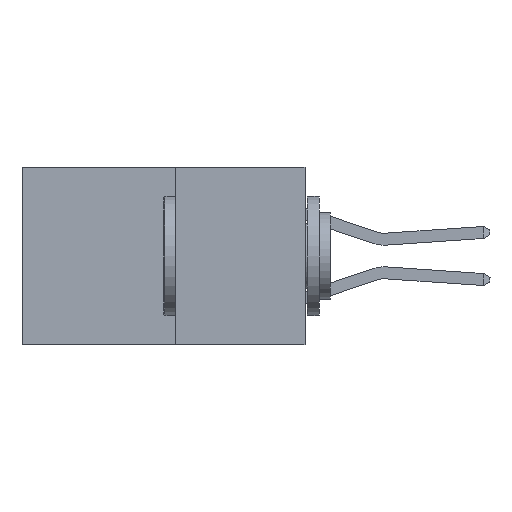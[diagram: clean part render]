
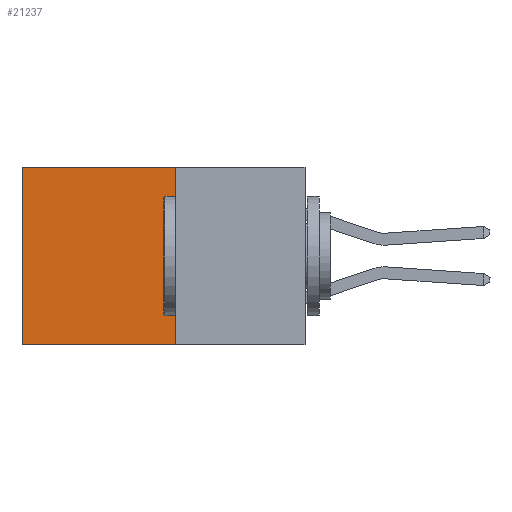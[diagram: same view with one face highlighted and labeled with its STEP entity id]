
A CAD part, left-side view. The second image highlights one B-rep face of the part: STEP entity #21237.
In plain terms, the highlighted planar face has unit normal (-1, 0, 0).
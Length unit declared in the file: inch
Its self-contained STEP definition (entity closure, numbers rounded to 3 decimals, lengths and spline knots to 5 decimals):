
#1875 = ORIENTED_EDGE ( 'NONE', *, *, #5821, .T. ) ;
#1978 = DIRECTION ( 'NONE',  ( 0., 1., 0. ) ) ;
#2347 = CARTESIAN_POINT ( 'NONE',  ( 0.277, 0.59, -0.37 ) ) ;
#3341 = CARTESIAN_POINT ( 'NONE',  ( 0.277, 0.27, -0.37 ) ) ;
#3669 = VECTOR ( 'NONE', #21332, 39.37008 ) ;
#4539 = CARTESIAN_POINT ( 'NONE',  ( 0.277, 0.27, 0. ) ) ;
#5821 = EDGE_CURVE ( 'NONE', #18430, #14609, #11507, .T. ) ;
#5999 = CARTESIAN_POINT ( 'NONE',  ( 0.277, 0.27, -0.37 ) ) ;
#6032 = CARTESIAN_POINT ( 'NONE',  ( 0.277, 0.27, 0. ) ) ;
#7014 = FACE_OUTER_BOUND ( 'NONE', #12548, .T. ) ;
#8578 = PLANE ( 'NONE',  #15461 ) ;
#10175 = ORIENTED_EDGE ( 'NONE', *, *, #31992, .F. ) ;
#10343 = DIRECTION ( 'NONE',  ( 0., 0., -1. ) ) ;
#10533 = CARTESIAN_POINT ( 'NONE',  ( 0.277, 0.59, -0.37 ) ) ;
#10914 = ORIENTED_EDGE ( 'NONE', *, *, #27633, .T. ) ;
#11176 = DIRECTION ( 'NONE',  ( 0., 0., -1. ) ) ;
#11507 = LINE ( 'NONE', #10533, #12329 ) ;
#12329 = VECTOR ( 'NONE', #10343, 39.37008 ) ;
#12548 = EDGE_LOOP ( 'NONE', ( #1875, #32816, #10175, #10914 ) ) ;
#12739 = DIRECTION ( 'NONE',  ( 0., 0., -1. ) ) ;
#13264 = VECTOR ( 'NONE', #1978, 39.37008 ) ;
#14609 = VERTEX_POINT ( 'NONE', #2347 ) ;
#15461 = AXIS2_PLACEMENT_3D ( 'NONE', #5999, #16242, #11176 ) ;
#16242 = DIRECTION ( 'NONE',  ( 1., 0., 0. ) ) ;
#18430 = VERTEX_POINT ( 'NONE', #27172 ) ;
#21237 = ADVANCED_FACE ( 'NONE', ( #7014 ), #8578, .F. ) ;
#21332 = DIRECTION ( 'NONE',  ( 0., 1., 0. ) ) ;
#22663 = VERTEX_POINT ( 'NONE', #6032 ) ;
#23397 = LINE ( 'NONE', #3341, #3669 ) ;
#25602 = CARTESIAN_POINT ( 'NONE',  ( 0.277, 0.27, -0.37 ) ) ;
#25870 = CARTESIAN_POINT ( 'NONE',  ( 0.277, 0.27, -0.37 ) ) ;
#26308 = LINE ( 'NONE', #25602, #32348 ) ;
#26997 = LINE ( 'NONE', #4539, #13264 ) ;
#27172 = CARTESIAN_POINT ( 'NONE',  ( 0.277, 0.59, 0. ) ) ;
#27633 = EDGE_CURVE ( 'NONE', #22663, #18430, #26997, .T. ) ;
#28521 = VERTEX_POINT ( 'NONE', #25870 ) ;
#31992 = EDGE_CURVE ( 'NONE', #22663, #28521, #26308, .T. ) ;
#32348 = VECTOR ( 'NONE', #12739, 39.37008 ) ;
#32816 = ORIENTED_EDGE ( 'NONE', *, *, #33200, .F. ) ;
#33200 = EDGE_CURVE ( 'NONE', #28521, #14609, #23397, .T. ) ;
